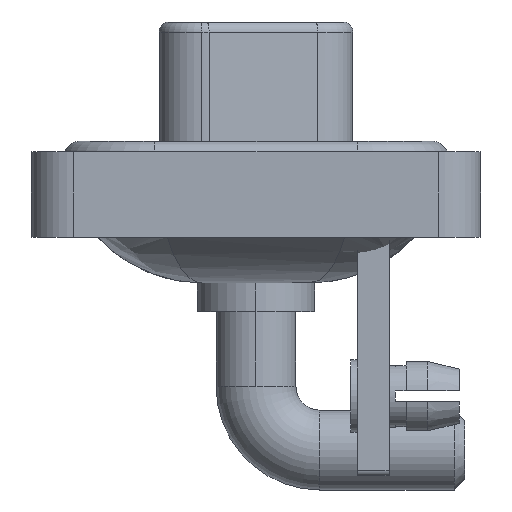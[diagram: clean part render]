
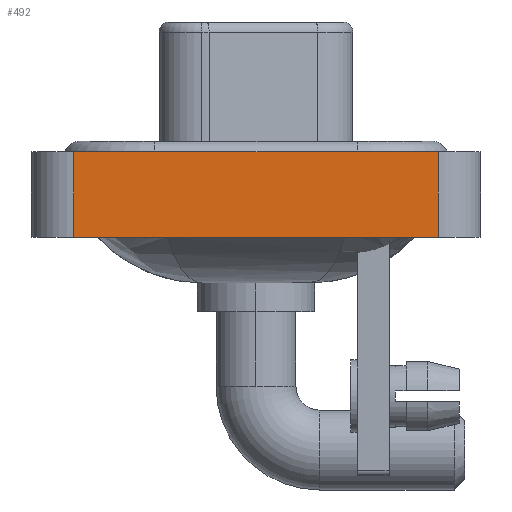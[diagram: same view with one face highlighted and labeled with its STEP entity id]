
A CAD part, left-side view. The second image highlights one B-rep face of the part: STEP entity #492.
In plain terms, the highlighted planar face has unit normal (-1, 0, 0).
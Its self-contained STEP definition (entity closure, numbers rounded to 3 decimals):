
#440 = VECTOR ( 'NONE', #17797, 1000. ) ;
#492 = ADVANCED_FACE ( 'NONE', ( #7653 ), #13964, .T. ) ;
#873 = LINE ( 'NONE', #9068, #13063 ) ;
#1021 = CARTESIAN_POINT ( 'NONE',  ( -7.35, 8.55, 0.4 ) ) ;
#2134 = ORIENTED_EDGE ( 'NONE', *, *, #6767, .F. ) ;
#3560 = LINE ( 'NONE', #15034, #8157 ) ;
#3665 = CARTESIAN_POINT ( 'NONE',  ( -7.35, 8.55, -3.6 ) ) ;
#4838 = DIRECTION ( 'NONE',  ( 0., 0., 1. ) ) ;
#5892 = CARTESIAN_POINT ( 'NONE',  ( -7.35, -8.55, -3.6 ) ) ;
#6424 = EDGE_LOOP ( 'NONE', ( #16673, #2134, #11392, #8655 ) ) ;
#6725 = EDGE_CURVE ( 'NONE', #9374, #8259, #14684, .T. ) ;
#6767 = EDGE_CURVE ( 'NONE', #16075, #19222, #14792, .T. ) ;
#7653 = FACE_OUTER_BOUND ( 'NONE', #6424, .T. ) ;
#7855 = DIRECTION ( 'NONE',  ( -1., 0., 0. ) ) ;
#8157 = VECTOR ( 'NONE', #9881, 1000. ) ;
#8259 = VERTEX_POINT ( 'NONE', #5892 ) ;
#8655 = ORIENTED_EDGE ( 'NONE', *, *, #6725, .T. ) ;
#8719 = VECTOR ( 'NONE', #11597, 1000. ) ;
#9068 = CARTESIAN_POINT ( 'NONE',  ( -7.35, -8.55, -3.6 ) ) ;
#9307 = EDGE_CURVE ( 'NONE', #9374, #16075, #3560, .T. ) ;
#9374 = VERTEX_POINT ( 'NONE', #3665 ) ;
#9881 = DIRECTION ( 'NONE',  ( 0., 0., 1. ) ) ;
#11392 = ORIENTED_EDGE ( 'NONE', *, *, #9307, .F. ) ;
#11597 = DIRECTION ( 'NONE',  ( 0., -1., 0. ) ) ;
#11797 = CARTESIAN_POINT ( 'NONE',  ( -7.35, -8.55, 0.4 ) ) ;
#12624 = CARTESIAN_POINT ( 'NONE',  ( -7.35, -8.55, -3.6 ) ) ;
#13063 = VECTOR ( 'NONE', #15364, 1000. ) ;
#13964 = PLANE ( 'NONE',  #17840 ) ;
#14285 = EDGE_CURVE ( 'NONE', #8259, #19222, #873, .T. ) ;
#14684 = LINE ( 'NONE', #16330, #8719 ) ;
#14792 = LINE ( 'NONE', #11797, #440 ) ;
#15034 = CARTESIAN_POINT ( 'NONE',  ( -7.35, 8.55, -3.6 ) ) ;
#15364 = DIRECTION ( 'NONE',  ( 0., 0., 1. ) ) ;
#16075 = VERTEX_POINT ( 'NONE', #1021 ) ;
#16330 = CARTESIAN_POINT ( 'NONE',  ( -7.35, -8.55, -3.6 ) ) ;
#16673 = ORIENTED_EDGE ( 'NONE', *, *, #14285, .T. ) ;
#17797 = DIRECTION ( 'NONE',  ( 0., -1., 0. ) ) ;
#17840 = AXIS2_PLACEMENT_3D ( 'NONE', #12624, #7855, #4838 ) ;
#19222 = VERTEX_POINT ( 'NONE', #19319 ) ;
#19319 = CARTESIAN_POINT ( 'NONE',  ( -7.35, -8.55, 0.4 ) ) ;
